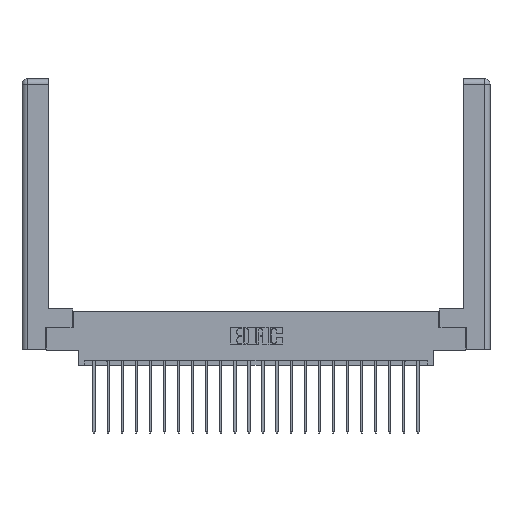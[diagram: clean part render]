
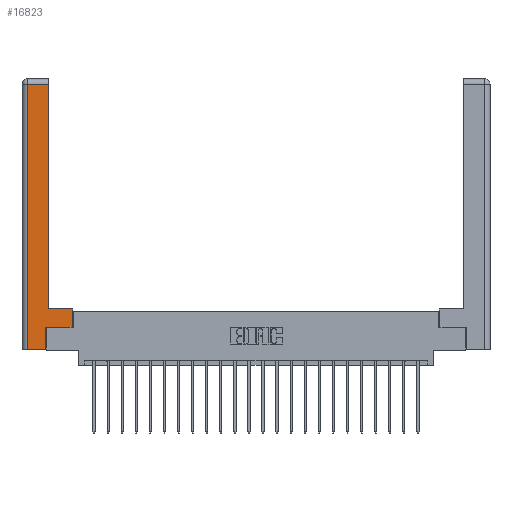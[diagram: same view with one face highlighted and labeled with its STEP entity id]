
A CAD part, top view. The second image highlights one B-rep face of the part: STEP entity #16823.
In plain terms, the highlighted planar face has unit normal (0, 0, 1).
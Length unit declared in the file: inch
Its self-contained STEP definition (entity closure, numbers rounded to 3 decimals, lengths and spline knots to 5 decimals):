
#50 = VERTEX_POINT ( 'NONE', #13789 ) ;
#817 = ORIENTED_EDGE ( 'NONE', *, *, #2437, .T. ) ;
#1643 = CARTESIAN_POINT ( 'NONE',  ( 0.295, 0.45, 0. ) ) ;
#1858 = CARTESIAN_POINT ( 'NONE',  ( 0.565, 0.245, 0. ) ) ;
#2097 = EDGE_CURVE ( 'NONE', #8153, #9086, #22041, .T. ) ;
#2221 = LINE ( 'NONE', #4200, #18000 ) ;
#2314 = VECTOR ( 'NONE', #8743, 39.37008 ) ;
#2420 = EDGE_LOOP ( 'NONE', ( #15972, #7674, #15039, #9925, #20645, #817, #13558, #13415 ) ) ;
#2437 = EDGE_CURVE ( 'NONE', #9258, #8372, #5361, .T. ) ;
#2998 = CARTESIAN_POINT ( 'NONE',  ( 0.565, 0.45, 0. ) ) ;
#3264 = LINE ( 'NONE', #21511, #23358 ) ;
#3281 = CARTESIAN_POINT ( 'NONE',  ( 0.265, 0., 0. ) ) ;
#3399 = DIRECTION ( 'NONE',  ( 0., -1., 0. ) ) ;
#3464 = DIRECTION ( 'NONE',  ( -1., 0., 0. ) ) ;
#3671 = CARTESIAN_POINT ( 'NONE',  ( 0.0615, 0., 0. ) ) ;
#3800 = EDGE_CURVE ( 'NONE', #22680, #4400, #20509, .T. ) ;
#4200 = CARTESIAN_POINT ( 'NONE',  ( 0.265, 0.245, 0. ) ) ;
#4400 = VERTEX_POINT ( 'NONE', #3671 ) ;
#5123 = CARTESIAN_POINT ( 'NONE',  ( 0.265, 0.245, 0. ) ) ;
#5361 = LINE ( 'NONE', #1858, #22849 ) ;
#5847 = CARTESIAN_POINT ( 'NONE',  ( 0.265, 0., 0. ) ) ;
#5938 = VECTOR ( 'NONE', #3464, 39.37008 ) ;
#6693 = DIRECTION ( 'NONE',  ( -1., 0., 0. ) ) ;
#7095 = CARTESIAN_POINT ( 'NONE',  ( 0.0615, 0., 0. ) ) ;
#7674 = ORIENTED_EDGE ( 'NONE', *, *, #22007, .T. ) ;
#7846 = AXIS2_PLACEMENT_3D ( 'NONE', #15952, #14043, #6693 ) ;
#8153 = VERTEX_POINT ( 'NONE', #2998 ) ;
#8372 = VERTEX_POINT ( 'NONE', #10536 ) ;
#8743 = DIRECTION ( 'NONE',  ( 1., 0., 0. ) ) ;
#9086 = VERTEX_POINT ( 'NONE', #23166 ) ;
#9258 = VERTEX_POINT ( 'NONE', #5123 ) ;
#9569 = VECTOR ( 'NONE', #19255, 39.37008 ) ;
#9925 = ORIENTED_EDGE ( 'NONE', *, *, #21501, .T. ) ;
#10536 = CARTESIAN_POINT ( 'NONE',  ( 0.565, 0.245, 0. ) ) ;
#10595 = FACE_OUTER_BOUND ( 'NONE', #2420, .T. ) ;
#12361 = EDGE_CURVE ( 'NONE', #8372, #8153, #3264, .T. ) ;
#13415 = ORIENTED_EDGE ( 'NONE', *, *, #2097, .T. ) ;
#13558 = ORIENTED_EDGE ( 'NONE', *, *, #12361, .T. ) ;
#13589 = CARTESIAN_POINT ( 'NONE',  ( 0.295, 3., 0. ) ) ;
#13648 = DIRECTION ( 'NONE',  ( -1., 0., 0. ) ) ;
#13789 = CARTESIAN_POINT ( 'NONE',  ( 0.295, 2.94, 0. ) ) ;
#14043 = DIRECTION ( 'NONE',  ( 0., 0., -1. ) ) ;
#15039 = ORIENTED_EDGE ( 'NONE', *, *, #3800, .T. ) ;
#15951 = EDGE_CURVE ( 'NONE', #17363, #9258, #2221, .T. ) ;
#15952 = CARTESIAN_POINT ( 'NONE',  ( 0., 0., 0. ) ) ;
#15972 = ORIENTED_EDGE ( 'NONE', *, *, #20013, .T. ) ;
#16823 = ADVANCED_FACE ( 'NONE', ( #10595 ), #17677, .F. ) ;
#17219 = LINE ( 'NONE', #17469, #17486 ) ;
#17363 = VERTEX_POINT ( 'NONE', #5847 ) ;
#17469 = CARTESIAN_POINT ( 'NONE',  ( 0.0615, 2.94, 0. ) ) ;
#17486 = VECTOR ( 'NONE', #13648, 39.37008 ) ;
#17677 = PLANE ( 'NONE',  #7846 ) ;
#18000 = VECTOR ( 'NONE', #22400, 39.37008 ) ;
#18931 = LINE ( 'NONE', #3281, #2314 ) ;
#19173 = CARTESIAN_POINT ( 'NONE',  ( 0.0615, 2.94, 0. ) ) ;
#19255 = DIRECTION ( 'NONE',  ( 0., 1., 0. ) ) ;
#20013 = EDGE_CURVE ( 'NONE', #9086, #50, #23055, .T. ) ;
#20509 = LINE ( 'NONE', #7095, #23688 ) ;
#20645 = ORIENTED_EDGE ( 'NONE', *, *, #15951, .T. ) ;
#21501 = EDGE_CURVE ( 'NONE', #4400, #17363, #18931, .T. ) ;
#21511 = CARTESIAN_POINT ( 'NONE',  ( 0.565, 0.45, 0. ) ) ;
#22007 = EDGE_CURVE ( 'NONE', #50, #22680, #17219, .T. ) ;
#22041 = LINE ( 'NONE', #1643, #5938 ) ;
#22135 = DIRECTION ( 'NONE',  ( 1., 0., 0. ) ) ;
#22400 = DIRECTION ( 'NONE',  ( 0., 1., 0. ) ) ;
#22680 = VERTEX_POINT ( 'NONE', #19173 ) ;
#22849 = VECTOR ( 'NONE', #22135, 39.37008 ) ;
#23055 = LINE ( 'NONE', #13589, #9569 ) ;
#23166 = CARTESIAN_POINT ( 'NONE',  ( 0.295, 0.45, 0. ) ) ;
#23358 = VECTOR ( 'NONE', #23360, 39.37008 ) ;
#23360 = DIRECTION ( 'NONE',  ( 0., 1., 0. ) ) ;
#23688 = VECTOR ( 'NONE', #3399, 39.37008 ) ;
